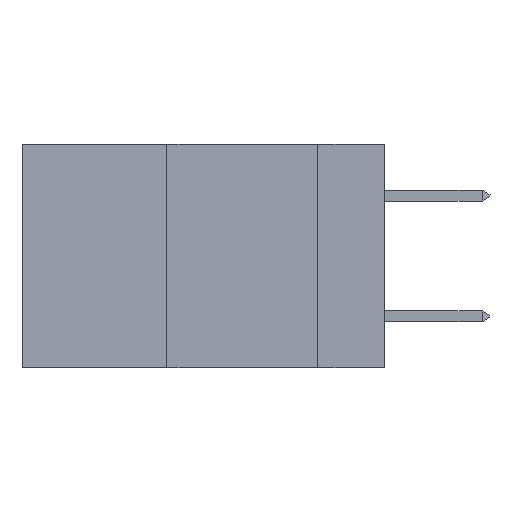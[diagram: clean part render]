
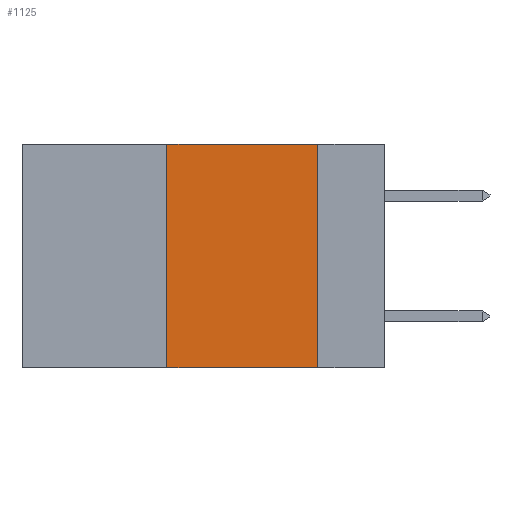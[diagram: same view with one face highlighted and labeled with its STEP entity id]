
A CAD part, left-side view. The second image highlights one B-rep face of the part: STEP entity #1125.
In plain terms, the highlighted planar face has unit normal (-1, 0, 0).
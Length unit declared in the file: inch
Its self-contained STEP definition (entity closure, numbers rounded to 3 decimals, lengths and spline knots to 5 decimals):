
#49 = ORIENTED_EDGE ( 'NONE', *, *, #5512, .T. ) ;
#948 = AXIS2_PLACEMENT_3D ( 'NONE', #9396, #5258, #2269 ) ;
#1036 = ORIENTED_EDGE ( 'NONE', *, *, #3358, .F. ) ;
#1050 = ORIENTED_EDGE ( 'NONE', *, *, #6640, .F. ) ;
#1125 = ADVANCED_FACE ( 'NONE', ( #6898 ), #9481, .F. ) ;
#1442 = LINE ( 'NONE', #6707, #3214 ) ;
#1509 = LINE ( 'NONE', #5753, #9193 ) ;
#1772 = DIRECTION ( 'NONE',  ( 0., -1., 0. ) ) ;
#2068 = VERTEX_POINT ( 'NONE', #8277 ) ;
#2070 = DIRECTION ( 'NONE',  ( 0., -1., 0. ) ) ;
#2262 = ORIENTED_EDGE ( 'NONE', *, *, #5264, .F. ) ;
#2269 = DIRECTION ( 'NONE',  ( 0., 0., -1. ) ) ;
#2664 = VERTEX_POINT ( 'NONE', #3846 ) ;
#3214 = VECTOR ( 'NONE', #9587, 39.37008 ) ;
#3358 = EDGE_CURVE ( 'NONE', #3617, #2068, #1442, .T. ) ;
#3439 = CARTESIAN_POINT ( 'NONE',  ( 0., 0.36, 0. ) ) ;
#3444 = VECTOR ( 'NONE', #1772, 39.37008 ) ;
#3571 = EDGE_LOOP ( 'NONE', ( #1036, #1050, #2262, #49 ) ) ;
#3617 = VERTEX_POINT ( 'NONE', #9576 ) ;
#3846 = CARTESIAN_POINT ( 'NONE',  ( 0., 0.36, -0.37 ) ) ;
#5258 = DIRECTION ( 'NONE',  ( 1., 0., 0. ) ) ;
#5264 = EDGE_CURVE ( 'NONE', #2664, #7133, #7399, .T. ) ;
#5409 = LINE ( 'NONE', #7045, #3444 ) ;
#5512 = EDGE_CURVE ( 'NONE', #2664, #2068, #1509, .T. ) ;
#5753 = CARTESIAN_POINT ( 'NONE',  ( 0., 0.6, -0.37 ) ) ;
#6640 = EDGE_CURVE ( 'NONE', #7133, #3617, #5409, .T. ) ;
#6707 = CARTESIAN_POINT ( 'NONE',  ( 0., 0.11, 0. ) ) ;
#6898 = FACE_OUTER_BOUND ( 'NONE', #3571, .T. ) ;
#7045 = CARTESIAN_POINT ( 'NONE',  ( 0., 0.6, 0. ) ) ;
#7133 = VERTEX_POINT ( 'NONE', #8955 ) ;
#7166 = VECTOR ( 'NONE', #8370, 39.37008 ) ;
#7399 = LINE ( 'NONE', #3439, #7166 ) ;
#8277 = CARTESIAN_POINT ( 'NONE',  ( 0., 0.11, -0.37 ) ) ;
#8370 = DIRECTION ( 'NONE',  ( 0., 0., 1. ) ) ;
#8955 = CARTESIAN_POINT ( 'NONE',  ( 0., 0.36, 0. ) ) ;
#9193 = VECTOR ( 'NONE', #2070, 39.37008 ) ;
#9396 = CARTESIAN_POINT ( 'NONE',  ( 0., 0.6, 0. ) ) ;
#9481 = PLANE ( 'NONE',  #948 ) ;
#9576 = CARTESIAN_POINT ( 'NONE',  ( 0., 0.11, 0. ) ) ;
#9587 = DIRECTION ( 'NONE',  ( 0., 0., -1. ) ) ;
